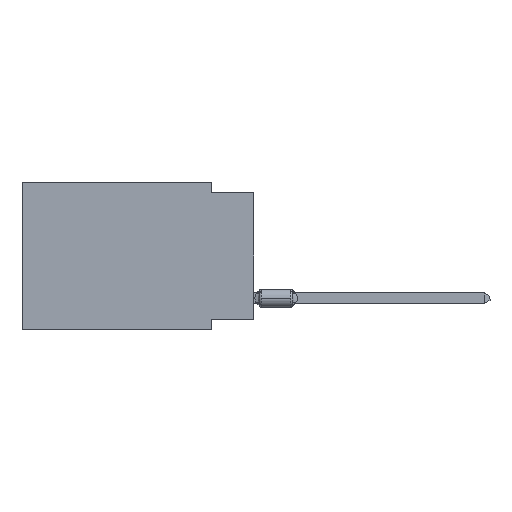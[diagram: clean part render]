
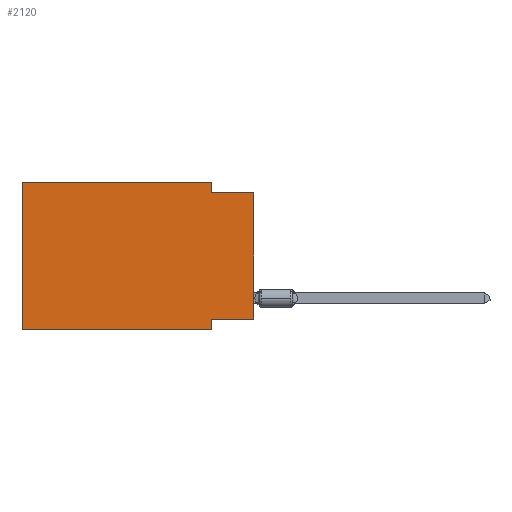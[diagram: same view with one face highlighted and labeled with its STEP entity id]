
A CAD part, left-side view. The second image highlights one B-rep face of the part: STEP entity #2120.
In plain terms, the highlighted planar face has unit normal (-1, 0, 0).
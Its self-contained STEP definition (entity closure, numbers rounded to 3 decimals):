
#82 = PLANE ( 'NONE',  #14298 ) ;
#354 = ORIENTED_EDGE ( 'NONE', *, *, #7261, .F. ) ;
#871 = CARTESIAN_POINT ( 'NONE',  ( 0., 0., -0.635 ) ) ;
#1040 = EDGE_CURVE ( 'NONE', #14472, #12628, #16286, .T. ) ;
#1838 = CARTESIAN_POINT ( 'NONE',  ( 0., 2.54, 0. ) ) ;
#2120 = ADVANCED_FACE ( 'NONE', ( #13702 ), #82, .F. ) ;
#2365 = CARTESIAN_POINT ( 'NONE',  ( 0., 13.97, -8.89 ) ) ;
#2494 = EDGE_LOOP ( 'NONE', ( #16302, #15914, #12742, #13330, #16921, #3219, #13963, #354 ) ) ;
#2671 = CARTESIAN_POINT ( 'NONE',  ( 0., 0., -0.635 ) ) ;
#3219 = ORIENTED_EDGE ( 'NONE', *, *, #6664, .T. ) ;
#3524 = LINE ( 'NONE', #1838, #5143 ) ;
#3824 = CARTESIAN_POINT ( 'NONE',  ( 0., 2.54, -8.89 ) ) ;
#4239 = DIRECTION ( 'NONE',  ( 0., -1., 0. ) ) ;
#5143 = VECTOR ( 'NONE', #6312, 1000. ) ;
#5415 = LINE ( 'NONE', #3824, #14095 ) ;
#6012 = LINE ( 'NONE', #2365, #12237 ) ;
#6119 = VERTEX_POINT ( 'NONE', #12916 ) ;
#6158 = DIRECTION ( 'NONE',  ( 1., 0., 0. ) ) ;
#6312 = DIRECTION ( 'NONE',  ( 0., 0., -1. ) ) ;
#6664 = EDGE_CURVE ( 'NONE', #18102, #6119, #6012, .T. ) ;
#7157 = CARTESIAN_POINT ( 'NONE',  ( 0., 0., -8.255 ) ) ;
#7261 = EDGE_CURVE ( 'NONE', #10437, #17316, #11079, .T. ) ;
#7762 = CARTESIAN_POINT ( 'NONE',  ( 0., 0., 0. ) ) ;
#8497 = LINE ( 'NONE', #8886, #9756 ) ;
#8886 = CARTESIAN_POINT ( 'NONE',  ( 0., 13.97, 0. ) ) ;
#9208 = CARTESIAN_POINT ( 'NONE',  ( 0., 13.97, 0. ) ) ;
#9253 = LINE ( 'NONE', #7762, #12625 ) ;
#9705 = EDGE_CURVE ( 'NONE', #12557, #14472, #3524, .T. ) ;
#9756 = VECTOR ( 'NONE', #4239, 1000. ) ;
#9870 = DIRECTION ( 'NONE',  ( 0., 0., -1. ) ) ;
#10437 = VERTEX_POINT ( 'NONE', #7157 ) ;
#10716 = DIRECTION ( 'NONE',  ( 0., 0., -1. ) ) ;
#10867 = DIRECTION ( 'NONE',  ( 0., 0., 1. ) ) ;
#11050 = DIRECTION ( 'NONE',  ( 0., 0., 1. ) ) ;
#11079 = LINE ( 'NONE', #12779, #15119 ) ;
#11389 = EDGE_CURVE ( 'NONE', #17316, #6119, #5415, .T. ) ;
#12033 = CARTESIAN_POINT ( 'NONE',  ( 0., 13.97, 0. ) ) ;
#12237 = VECTOR ( 'NONE', #13556, 1000. ) ;
#12557 = VERTEX_POINT ( 'NONE', #17367 ) ;
#12625 = VECTOR ( 'NONE', #11050, 1000. ) ;
#12628 = VERTEX_POINT ( 'NONE', #871 ) ;
#12742 = ORIENTED_EDGE ( 'NONE', *, *, #9705, .F. ) ;
#12779 = CARTESIAN_POINT ( 'NONE',  ( 0., 0., -8.255 ) ) ;
#12916 = CARTESIAN_POINT ( 'NONE',  ( 0., 2.54, -8.89 ) ) ;
#13214 = VECTOR ( 'NONE', #10867, 1000. ) ;
#13305 = CARTESIAN_POINT ( 'NONE',  ( 0., 2.54, -0.635 ) ) ;
#13330 = ORIENTED_EDGE ( 'NONE', *, *, #16470, .F. ) ;
#13442 = VERTEX_POINT ( 'NONE', #9208 ) ;
#13556 = DIRECTION ( 'NONE',  ( 0., -1., 0. ) ) ;
#13702 = FACE_OUTER_BOUND ( 'NONE', #2494, .T. ) ;
#13963 = ORIENTED_EDGE ( 'NONE', *, *, #11389, .F. ) ;
#14095 = VECTOR ( 'NONE', #9870, 1000. ) ;
#14296 = DIRECTION ( 'NONE',  ( 0., -1., 0. ) ) ;
#14298 = AXIS2_PLACEMENT_3D ( 'NONE', #12033, #6158, #10716 ) ;
#14347 = LINE ( 'NONE', #17132, #13214 ) ;
#14472 = VERTEX_POINT ( 'NONE', #13305 ) ;
#15119 = VECTOR ( 'NONE', #17244, 1000. ) ;
#15512 = VECTOR ( 'NONE', #14296, 1000. ) ;
#15538 = EDGE_CURVE ( 'NONE', #18102, #13442, #14347, .T. ) ;
#15695 = CARTESIAN_POINT ( 'NONE',  ( 0., 2.54, -8.255 ) ) ;
#15914 = ORIENTED_EDGE ( 'NONE', *, *, #1040, .F. ) ;
#16286 = LINE ( 'NONE', #2671, #15512 ) ;
#16302 = ORIENTED_EDGE ( 'NONE', *, *, #16704, .T. ) ;
#16470 = EDGE_CURVE ( 'NONE', #13442, #12557, #8497, .T. ) ;
#16704 = EDGE_CURVE ( 'NONE', #10437, #12628, #9253, .T. ) ;
#16921 = ORIENTED_EDGE ( 'NONE', *, *, #15538, .F. ) ;
#17132 = CARTESIAN_POINT ( 'NONE',  ( 0., 13.97, 0. ) ) ;
#17243 = CARTESIAN_POINT ( 'NONE',  ( 0., 13.97, -8.89 ) ) ;
#17244 = DIRECTION ( 'NONE',  ( 0., 1., 0. ) ) ;
#17316 = VERTEX_POINT ( 'NONE', #15695 ) ;
#17367 = CARTESIAN_POINT ( 'NONE',  ( 0., 2.54, 0. ) ) ;
#18102 = VERTEX_POINT ( 'NONE', #17243 ) ;
